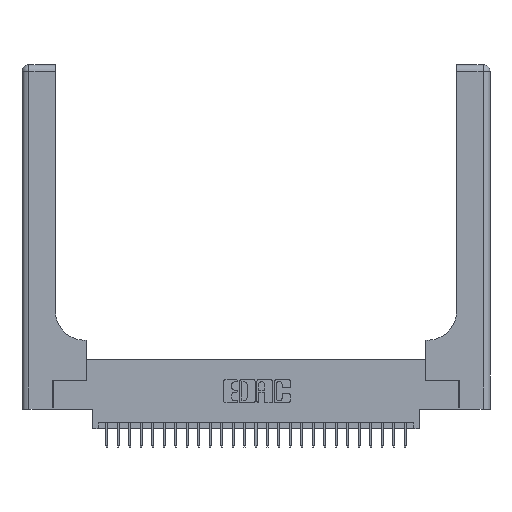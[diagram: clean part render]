
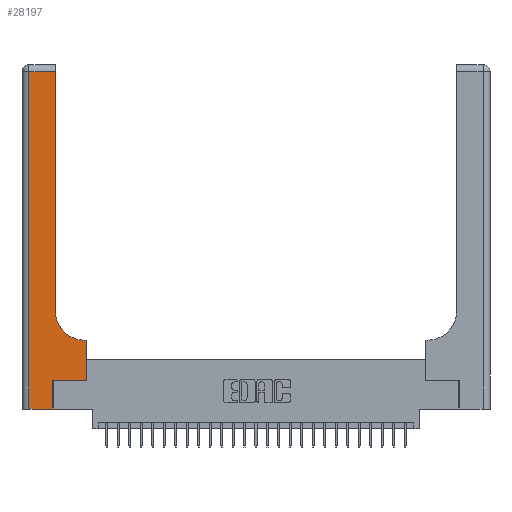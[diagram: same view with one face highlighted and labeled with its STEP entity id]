
A CAD part, top view. The second image highlights one B-rep face of the part: STEP entity #28197.
In plain terms, the highlighted planar face has unit normal (0, 0, 1).
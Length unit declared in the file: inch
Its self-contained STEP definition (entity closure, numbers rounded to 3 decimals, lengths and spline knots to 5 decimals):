
#41 = DIRECTION ( 'NONE',  ( 1., 0., 0. ) ) ;
#117 = DIRECTION ( 'NONE',  ( 1., 0., 0. ) ) ;
#806 = AXIS2_PLACEMENT_3D ( 'NONE', #11438, #26644, #13620 ) ;
#1812 = LINE ( 'NONE', #17229, #24664 ) ;
#2230 = EDGE_CURVE ( 'NONE', #11916, #10350, #17308, .T. ) ;
#4261 = LINE ( 'NONE', #19796, #15525 ) ;
#4739 = ORIENTED_EDGE ( 'NONE', *, *, #2230, .T. ) ;
#4751 = CARTESIAN_POINT ( 'NONE',  ( 0.5585, 0.6, 0.37 ) ) ;
#4860 = VERTEX_POINT ( 'NONE', #4751 ) ;
#5359 = DIRECTION ( 'NONE',  ( 0., -1., 0. ) ) ;
#6065 = DIRECTION ( 'NONE',  ( 0., 1., 0. ) ) ;
#6103 = AXIS2_PLACEMENT_3D ( 'NONE', #26565, #13547, #41 ) ;
#6939 = CARTESIAN_POINT ( 'NONE',  ( 0.06, 2.94, 0.37 ) ) ;
#7352 = EDGE_CURVE ( 'NONE', #23512, #24542, #9217, .T. ) ;
#7834 = VECTOR ( 'NONE', #14884, 39.37008 ) ;
#8262 = CARTESIAN_POINT ( 'NONE',  ( 0.269, 0., 0.37 ) ) ;
#8875 = CARTESIAN_POINT ( 'NONE',  ( 0.06, 0., 0.37 ) ) ;
#8900 = FACE_OUTER_BOUND ( 'NONE', #19555, .T. ) ;
#9217 = LINE ( 'NONE', #28262, #15103 ) ;
#9285 = ORIENTED_EDGE ( 'NONE', *, *, #7352, .T. ) ;
#9909 = ORIENTED_EDGE ( 'NONE', *, *, #13912, .T. ) ;
#10059 = CARTESIAN_POINT ( 'NONE',  ( 0.2915, 2.94, 0.37 ) ) ;
#10319 = ORIENTED_EDGE ( 'NONE', *, *, #24129, .T. ) ;
#10350 = VERTEX_POINT ( 'NONE', #15902 ) ;
#10574 = CARTESIAN_POINT ( 'NONE',  ( 0.5415, 0.6, 0.37 ) ) ;
#11313 = EDGE_CURVE ( 'NONE', #25559, #13927, #26171, .T. ) ;
#11438 = CARTESIAN_POINT ( 'NONE',  ( 0., 3., 0.37 ) ) ;
#11916 = VERTEX_POINT ( 'NONE', #10574 ) ;
#12533 = VERTEX_POINT ( 'NONE', #19057 ) ;
#12851 = VECTOR ( 'NONE', #117, 39.37008 ) ;
#13208 = LINE ( 'NONE', #18737, #24155 ) ;
#13547 = DIRECTION ( 'NONE',  ( 0., 0., -1. ) ) ;
#13620 = DIRECTION ( 'NONE',  ( -1., 0., 0. ) ) ;
#13744 = ORIENTED_EDGE ( 'NONE', *, *, #13953, .T. ) ;
#13885 = VERTEX_POINT ( 'NONE', #21298 ) ;
#13912 = EDGE_CURVE ( 'NONE', #13927, #12533, #14458, .T. ) ;
#13927 = VERTEX_POINT ( 'NONE', #8262 ) ;
#13953 = EDGE_CURVE ( 'NONE', #10350, #23512, #1812, .T. ) ;
#14074 = EDGE_CURVE ( 'NONE', #13885, #4860, #4261, .T. ) ;
#14458 = LINE ( 'NONE', #25683, #7834 ) ;
#14884 = DIRECTION ( 'NONE',  ( 0., 1., 0. ) ) ;
#15103 = VECTOR ( 'NONE', #21829, 39.37008 ) ;
#15525 = VECTOR ( 'NONE', #28384, 39.37008 ) ;
#15806 = CARTESIAN_POINT ( 'NONE',  ( 0.269, 0.25, 0.37 ) ) ;
#15902 = CARTESIAN_POINT ( 'NONE',  ( 0.2915, 0.85, 0.37 ) ) ;
#15992 = CARTESIAN_POINT ( 'NONE',  ( 0.2915, 0.6, 0.37 ) ) ;
#17229 = CARTESIAN_POINT ( 'NONE',  ( 0.2915, 3., 0.37 ) ) ;
#17308 = CIRCLE ( 'NONE', #6103, 0.25 ) ;
#18030 = PLANE ( 'NONE',  #806 ) ;
#18082 = ORIENTED_EDGE ( 'NONE', *, *, #14074, .T. ) ;
#18204 = DIRECTION ( 'NONE',  ( -1., 0., 0. ) ) ;
#18737 = CARTESIAN_POINT ( 'NONE',  ( 0.06, 3., 0.37 ) ) ;
#18768 = LINE ( 'NONE', #15806, #12851 ) ;
#19057 = CARTESIAN_POINT ( 'NONE',  ( 0.269, 0.25, 0.37 ) ) ;
#19555 = EDGE_LOOP ( 'NONE', ( #13744, #9285, #10319, #26668, #9909, #20797, #18082, #27797, #4739 ) ) ;
#19796 = CARTESIAN_POINT ( 'NONE',  ( 0.5585, 0.25, 0.37 ) ) ;
#20797 = ORIENTED_EDGE ( 'NONE', *, *, #25096, .T. ) ;
#21298 = CARTESIAN_POINT ( 'NONE',  ( 0.5585, 0.25, 0.37 ) ) ;
#21829 = DIRECTION ( 'NONE',  ( -1., 0., 0. ) ) ;
#23137 = LINE ( 'NONE', #15992, #28148 ) ;
#23512 = VERTEX_POINT ( 'NONE', #10059 ) ;
#24129 = EDGE_CURVE ( 'NONE', #24542, #25559, #13208, .T. ) ;
#24155 = VECTOR ( 'NONE', #5359, 39.37008 ) ;
#24542 = VERTEX_POINT ( 'NONE', #6939 ) ;
#24664 = VECTOR ( 'NONE', #6065, 39.37008 ) ;
#25096 = EDGE_CURVE ( 'NONE', #12533, #13885, #18768, .T. ) ;
#25134 = EDGE_CURVE ( 'NONE', #4860, #11916, #23137, .T. ) ;
#25388 = CARTESIAN_POINT ( 'NONE',  ( 0., 0., 0.37 ) ) ;
#25497 = VECTOR ( 'NONE', #27528, 39.37008 ) ;
#25559 = VERTEX_POINT ( 'NONE', #8875 ) ;
#25683 = CARTESIAN_POINT ( 'NONE',  ( 0.269, 0., 0.37 ) ) ;
#26171 = LINE ( 'NONE', #25388, #25497 ) ;
#26565 = CARTESIAN_POINT ( 'NONE',  ( 0.5415, 0.85, 0.37 ) ) ;
#26644 = DIRECTION ( 'NONE',  ( 0., 0., -1. ) ) ;
#26668 = ORIENTED_EDGE ( 'NONE', *, *, #11313, .T. ) ;
#27528 = DIRECTION ( 'NONE',  ( 1., 0., 0. ) ) ;
#27797 = ORIENTED_EDGE ( 'NONE', *, *, #25134, .T. ) ;
#28148 = VECTOR ( 'NONE', #18204, 39.37008 ) ;
#28197 = ADVANCED_FACE ( 'NONE', ( #8900 ), #18030, .F. ) ;
#28262 = CARTESIAN_POINT ( 'NONE',  ( 0., 2.94, 0.37 ) ) ;
#28384 = DIRECTION ( 'NONE',  ( 0., 1., 0. ) ) ;
